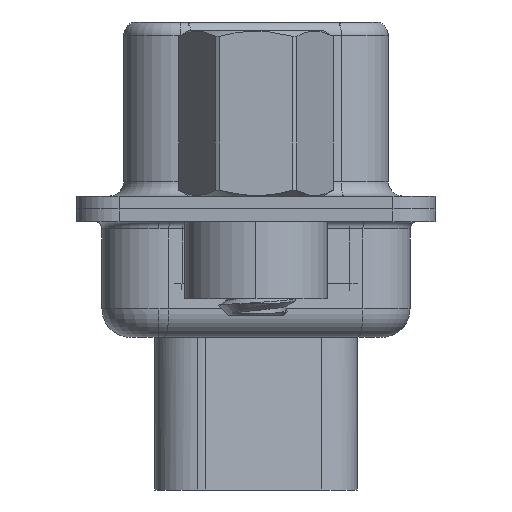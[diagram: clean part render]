
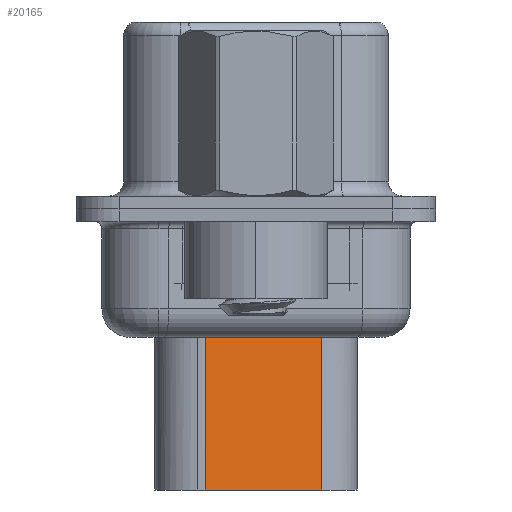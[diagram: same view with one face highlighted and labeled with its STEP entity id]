
A CAD part, left-side view. The second image highlights one B-rep face of the part: STEP entity #20165.
In plain terms, the highlighted planar face has unit normal (-0.985, -0.174, 0).
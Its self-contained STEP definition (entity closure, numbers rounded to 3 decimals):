
#1443 = VERTEX_POINT ( 'NONE', #26580 ) ;
#1704 = LINE ( 'NONE', #31718, #4247 ) ;
#3045 = VECTOR ( 'NONE', #4338, 1000. ) ;
#3993 = VERTEX_POINT ( 'NONE', #23282 ) ;
#4247 = VECTOR ( 'NONE', #11640, 1000. ) ;
#4338 = DIRECTION ( 'NONE',  ( -0.174, 0.985, 0. ) ) ;
#6396 = CARTESIAN_POINT ( 'NONE',  ( 4.524, 1.78, -3.1 ) ) ;
#6884 = EDGE_CURVE ( 'NONE', #15494, #26337, #9292, .T. ) ;
#7962 = CARTESIAN_POINT ( 'NONE',  ( 5.243, -2.3, -3.1 ) ) ;
#9292 = LINE ( 'NONE', #19871, #3045 ) ;
#11133 = VECTOR ( 'NONE', #30679, 1000. ) ;
#11475 = ORIENTED_EDGE ( 'NONE', *, *, #32500, .F. ) ;
#11640 = DIRECTION ( 'NONE',  ( -0.174, 0.985, 0. ) ) ;
#11835 = LINE ( 'NONE', #6396, #25415 ) ;
#12112 = FACE_OUTER_BOUND ( 'NONE', #17769, .T. ) ;
#12767 = CARTESIAN_POINT ( 'NONE',  ( 5.243, -2.3, -3.975 ) ) ;
#15494 = VERTEX_POINT ( 'NONE', #12767 ) ;
#15909 = CARTESIAN_POINT ( 'NONE',  ( 4.524, 1.78, -3.975 ) ) ;
#16313 = DIRECTION ( 'NONE',  ( 0., 0., -1. ) ) ;
#17769 = EDGE_LOOP ( 'NONE', ( #11475, #24943, #29103, #23541 ) ) ;
#19871 = CARTESIAN_POINT ( 'NONE',  ( 4.353, 2.749, -3.975 ) ) ;
#20165 = ADVANCED_FACE ( 'NONE', ( #12112 ), #27205, .T. ) ;
#20534 = LINE ( 'NONE', #7962, #11133 ) ;
#23282 = CARTESIAN_POINT ( 'NONE',  ( 4.524, 1.78, -9.85 ) ) ;
#23541 = ORIENTED_EDGE ( 'NONE', *, *, #28481, .F. ) ;
#24885 = DIRECTION ( 'NONE',  ( 0.174, -0.985, 0. ) ) ;
#24943 = ORIENTED_EDGE ( 'NONE', *, *, #6884, .T. ) ;
#25415 = VECTOR ( 'NONE', #16313, 1000. ) ;
#26337 = VERTEX_POINT ( 'NONE', #15909 ) ;
#26580 = CARTESIAN_POINT ( 'NONE',  ( 5.243, -2.3, -9.85 ) ) ;
#27205 = PLANE ( 'NONE',  #28166 ) ;
#27867 = DIRECTION ( 'NONE',  ( -0.985, -0.174, 0. ) ) ;
#28166 = AXIS2_PLACEMENT_3D ( 'NONE', #30028, #27867, #24885 ) ;
#28302 = EDGE_CURVE ( 'NONE', #26337, #3993, #11835, .T. ) ;
#28481 = EDGE_CURVE ( 'NONE', #1443, #3993, #1704, .T. ) ;
#29103 = ORIENTED_EDGE ( 'NONE', *, *, #28302, .T. ) ;
#30028 = CARTESIAN_POINT ( 'NONE',  ( 4.524, 1.78, -3.1 ) ) ;
#30679 = DIRECTION ( 'NONE',  ( 0., 0., -1. ) ) ;
#31718 = CARTESIAN_POINT ( 'NONE',  ( 4.524, 1.78, -9.85 ) ) ;
#32500 = EDGE_CURVE ( 'NONE', #15494, #1443, #20534, .T. ) ;
